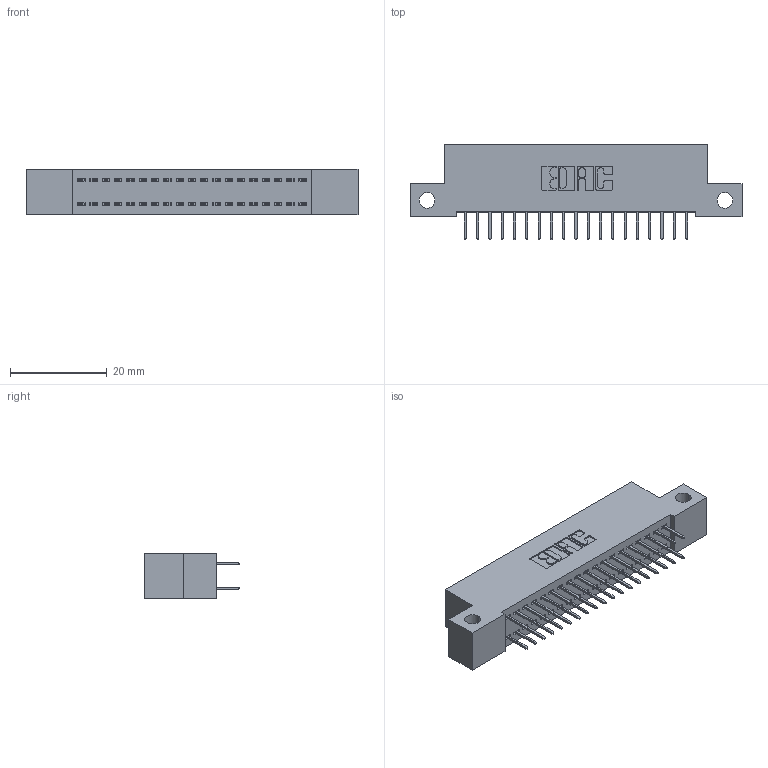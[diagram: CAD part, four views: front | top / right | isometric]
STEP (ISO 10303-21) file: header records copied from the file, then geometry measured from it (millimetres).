
FILE_DESCRIPTION (( 'STEP AP203' ), '1' );
FILE_NAME ('342-038-524-212.STEP', '2018-08-11T22:09:59', ( '' ), ( '' ), 'SwSTEP 2.0', 'SolidWorks 2016', '' );
FILE_SCHEMA (( 'CONFIG_CONTROL_DESIGN' ));
Length unit declared in the file: inch
Products named in the file (3): 342 Part_Side Mount; 345-292-001_345-293-124; 342-038-524-212
Assembly tree (39 placements, depth 2):
  342-038-524-212
    342 Part_Side Mount
    345-292-001_345-293-124  x38
Bounding box: 68.58 x 19.69 x 9.4 mm (x, y, z)
Volume: 5921.6 mm3; surface area: 8762.8 mm2
Topology: 39 solids, 39 shells, 2238 faces, 6341 edges, 4074 vertices
Faces by surface type: plane 1662, cylinder 576
Entity records: 15143 total; most frequent: CARTESIAN_POINT 2534, ORIENTED_EDGE 2470, DIRECTION 2207, EDGE_CURVE 1235, LINE 1111, VECTOR 1111, VERTEX_POINT 818, AXIS2_PLACEMENT_3D 548
